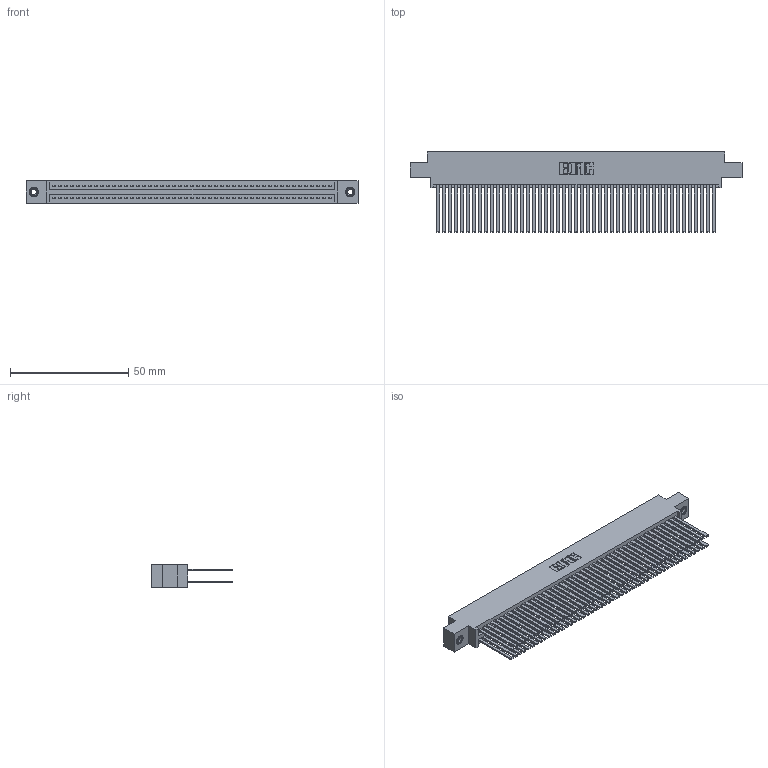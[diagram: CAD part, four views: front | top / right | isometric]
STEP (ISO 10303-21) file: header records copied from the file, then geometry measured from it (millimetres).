
FILE_DESCRIPTION (( 'STEP AP203' ), '1' );
FILE_NAME ('345-094-544-808.STEP', '2019-11-02T05:17:11', ( '' ), ( '' ), 'SwSTEP 2.0', 'SolidWorks 2016', '' );
FILE_SCHEMA (( 'CONFIG_CONTROL_DESIGN' ));
Length unit declared in the file: inch
Products named in the file (4): 345 Part_0.170 Offset - 0.156 Dia-TI; 345-094-544-808; 345-250-001_345-250-003-102; 345-292-001_345-293-144
Assembly tree (97 placements, depth 2):
  345-094-544-808
    345 Part_0.170 Offset - 0.156 Dia-TI
    345-292-001_345-293-144  x94
    345-250-001_345-250-003-102  x2
Bounding box: 140.59 x 33.96 x 9.4 mm (x, y, z)
Volume: 14901.2 mm3; surface area: 26142.3 mm2
Topology: 97 solids, 97 shells, 4326 faces, 12803 edges, 8402 vertices
Faces by surface type: plane 2842, cylinder 1468, cone 12, torus 4
Entity records: 37338 total; most frequent: CARTESIAN_POINT 6235, ORIENTED_EDGE 6162, DIRECTION 5515, EDGE_CURVE 3081, VECTOR 2745, LINE 2745, VERTEX_POINT 2048, AXIS2_PLACEMENT_3D 1385
